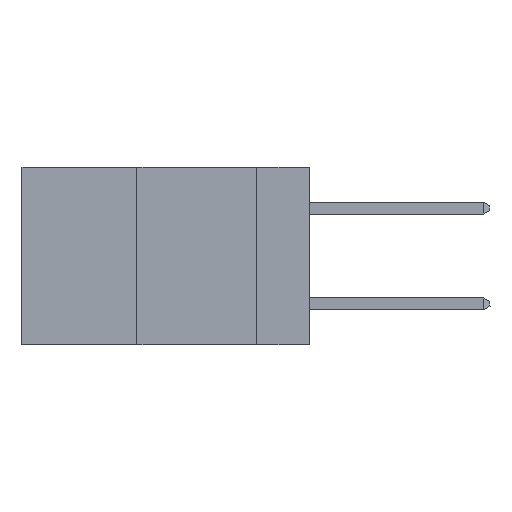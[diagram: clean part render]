
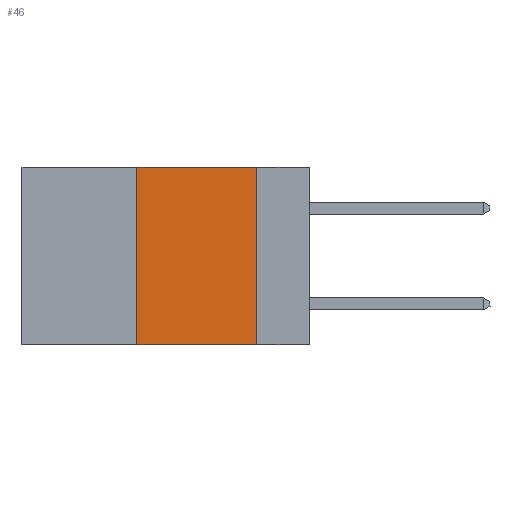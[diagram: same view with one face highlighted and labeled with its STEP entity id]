
A CAD part, left-side view. The second image highlights one B-rep face of the part: STEP entity #46.
In plain terms, the highlighted planar face has unit normal (-1, 0, 0).
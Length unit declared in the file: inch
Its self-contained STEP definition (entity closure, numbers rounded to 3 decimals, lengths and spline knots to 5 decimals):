
#3 = EDGE_CURVE ( 'NONE', #9205, #5146, #14956, .T. ) ;
#46 = ADVANCED_FACE ( 'NONE', ( #6069 ), #16350, .F. ) ;
#376 = VERTEX_POINT ( 'NONE', #15901 ) ;
#1616 = ORIENTED_EDGE ( 'NONE', *, *, #18294, .F. ) ;
#3162 = CARTESIAN_POINT ( 'NONE',  ( 0., 0.36, -0.37 ) ) ;
#3286 = VECTOR ( 'NONE', #10615, 39.37008 ) ;
#3500 = AXIS2_PLACEMENT_3D ( 'NONE', #8566, #16276, #16233 ) ;
#3671 = LINE ( 'NONE', #15573, #10044 ) ;
#4175 = CARTESIAN_POINT ( 'NONE',  ( 0., 0.11, -0.37 ) ) ;
#5146 = VERTEX_POINT ( 'NONE', #13451 ) ;
#5686 = ORIENTED_EDGE ( 'NONE', *, *, #3, .F. ) ;
#5983 = EDGE_CURVE ( 'NONE', #9205, #8986, #16584, .T. ) ;
#6069 = FACE_OUTER_BOUND ( 'NONE', #13119, .T. ) ;
#7477 = CARTESIAN_POINT ( 'NONE',  ( 0., 0.36, 0. ) ) ;
#8244 = DIRECTION ( 'NONE',  ( 0., 0., 1. ) ) ;
#8566 = CARTESIAN_POINT ( 'NONE',  ( 0., 0.6, 0. ) ) ;
#8986 = VERTEX_POINT ( 'NONE', #4175 ) ;
#9072 = ORIENTED_EDGE ( 'NONE', *, *, #10859, .F. ) ;
#9205 = VERTEX_POINT ( 'NONE', #3162 ) ;
#10044 = VECTOR ( 'NONE', #14028, 39.37008 ) ;
#10615 = DIRECTION ( 'NONE',  ( 0., -1., 0. ) ) ;
#10736 = VECTOR ( 'NONE', #8244, 39.37008 ) ;
#10859 = EDGE_CURVE ( 'NONE', #376, #8986, #3671, .T. ) ;
#12384 = CARTESIAN_POINT ( 'NONE',  ( 0., 0.6, -0.37 ) ) ;
#12474 = VECTOR ( 'NONE', #13978, 39.37008 ) ;
#13119 = EDGE_LOOP ( 'NONE', ( #9072, #1616, #5686, #13321 ) ) ;
#13321 = ORIENTED_EDGE ( 'NONE', *, *, #5983, .T. ) ;
#13451 = CARTESIAN_POINT ( 'NONE',  ( 0., 0.36, 0. ) ) ;
#13978 = DIRECTION ( 'NONE',  ( 0., -1., 0. ) ) ;
#14028 = DIRECTION ( 'NONE',  ( 0., 0., -1. ) ) ;
#14956 = LINE ( 'NONE', #7477, #10736 ) ;
#15335 = LINE ( 'NONE', #19888, #3286 ) ;
#15573 = CARTESIAN_POINT ( 'NONE',  ( 0., 0.11, 0. ) ) ;
#15901 = CARTESIAN_POINT ( 'NONE',  ( 0., 0.11, 0. ) ) ;
#16233 = DIRECTION ( 'NONE',  ( 0., 0., -1. ) ) ;
#16276 = DIRECTION ( 'NONE',  ( 1., 0., 0. ) ) ;
#16350 = PLANE ( 'NONE',  #3500 ) ;
#16584 = LINE ( 'NONE', #12384, #12474 ) ;
#18294 = EDGE_CURVE ( 'NONE', #5146, #376, #15335, .T. ) ;
#19888 = CARTESIAN_POINT ( 'NONE',  ( 0., 0.6, 0. ) ) ;
